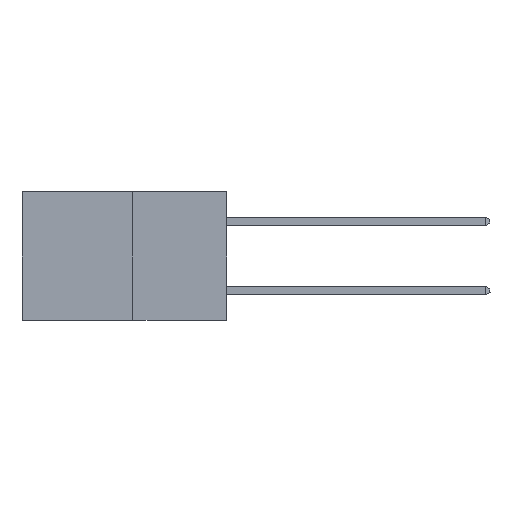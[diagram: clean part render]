
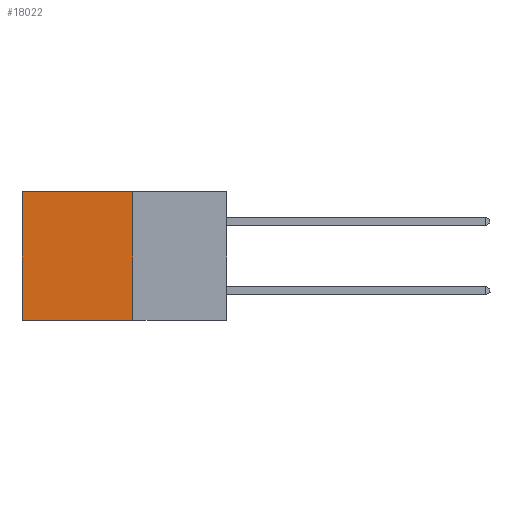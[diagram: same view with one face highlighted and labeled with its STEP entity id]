
A CAD part, left-side view. The second image highlights one B-rep face of the part: STEP entity #18022.
In plain terms, the highlighted planar face has unit normal (-1, 0, 0).
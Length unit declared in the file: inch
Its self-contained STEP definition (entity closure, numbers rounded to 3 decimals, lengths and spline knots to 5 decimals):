
#590 = FACE_OUTER_BOUND ( 'NONE', #11545, .T. ) ;
#1834 = VERTEX_POINT ( 'NONE', #18203 ) ;
#2158 = CARTESIAN_POINT ( 'NONE',  ( 0.277, 0.27, -0.37 ) ) ;
#2697 = VECTOR ( 'NONE', #7230, 39.37008 ) ;
#2786 = ORIENTED_EDGE ( 'NONE', *, *, #7210, .F. ) ;
#3764 = LINE ( 'NONE', #19265, #8458 ) ;
#3909 = VERTEX_POINT ( 'NONE', #9286 ) ;
#4207 = DIRECTION ( 'NONE',  ( 0., 0., -1. ) ) ;
#5300 = CARTESIAN_POINT ( 'NONE',  ( 0.277, 0.59, -0.37 ) ) ;
#5305 = EDGE_CURVE ( 'NONE', #20748, #5873, #20889, .T. ) ;
#5873 = VERTEX_POINT ( 'NONE', #15102 ) ;
#6187 = VECTOR ( 'NONE', #17468, 39.37008 ) ;
#6962 = CARTESIAN_POINT ( 'NONE',  ( 0.277, 0.59, 0. ) ) ;
#7210 = EDGE_CURVE ( 'NONE', #1834, #3909, #3764, .T. ) ;
#7230 = DIRECTION ( 'NONE',  ( 0., 1., 0. ) ) ;
#8458 = VECTOR ( 'NONE', #23126, 39.37008 ) ;
#9286 = CARTESIAN_POINT ( 'NONE',  ( 0.277, 0.27, -0.37 ) ) ;
#9314 = DIRECTION ( 'NONE',  ( 0., 0., -1. ) ) ;
#11545 = EDGE_LOOP ( 'NONE', ( #20488, #16193, #2786, #16606 ) ) ;
#12400 = EDGE_CURVE ( 'NONE', #3909, #5873, #18568, .T. ) ;
#15102 = CARTESIAN_POINT ( 'NONE',  ( 0.277, 0.59, -0.37 ) ) ;
#16092 = AXIS2_PLACEMENT_3D ( 'NONE', #2158, #16104, #4207 ) ;
#16104 = DIRECTION ( 'NONE',  ( 1., 0., 0. ) ) ;
#16193 = ORIENTED_EDGE ( 'NONE', *, *, #12400, .F. ) ;
#16606 = ORIENTED_EDGE ( 'NONE', *, *, #25224, .T. ) ;
#16728 = LINE ( 'NONE', #21283, #6187 ) ;
#17114 = CARTESIAN_POINT ( 'NONE',  ( 0.277, 0.27, -0.37 ) ) ;
#17468 = DIRECTION ( 'NONE',  ( 0., 1., 0. ) ) ;
#18022 = ADVANCED_FACE ( 'NONE', ( #590 ), #21903, .F. ) ;
#18203 = CARTESIAN_POINT ( 'NONE',  ( 0.277, 0.27, 0. ) ) ;
#18568 = LINE ( 'NONE', #17114, #2697 ) ;
#19265 = CARTESIAN_POINT ( 'NONE',  ( 0.277, 0.27, -0.37 ) ) ;
#20285 = VECTOR ( 'NONE', #9314, 39.37008 ) ;
#20488 = ORIENTED_EDGE ( 'NONE', *, *, #5305, .T. ) ;
#20748 = VERTEX_POINT ( 'NONE', #6962 ) ;
#20889 = LINE ( 'NONE', #5300, #20285 ) ;
#21283 = CARTESIAN_POINT ( 'NONE',  ( 0.277, 0.27, 0. ) ) ;
#21903 = PLANE ( 'NONE',  #16092 ) ;
#23126 = DIRECTION ( 'NONE',  ( 0., 0., -1. ) ) ;
#25224 = EDGE_CURVE ( 'NONE', #1834, #20748, #16728, .T. ) ;
